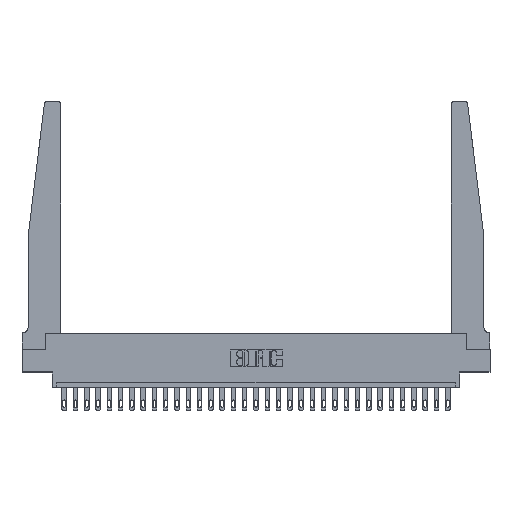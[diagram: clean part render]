
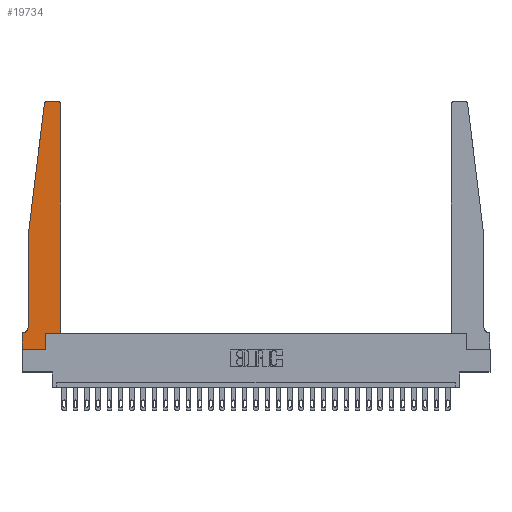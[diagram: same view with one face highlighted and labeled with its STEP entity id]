
A CAD part, top view. The second image highlights one B-rep face of the part: STEP entity #19734.
In plain terms, the highlighted planar face has unit normal (0, 0, 1).
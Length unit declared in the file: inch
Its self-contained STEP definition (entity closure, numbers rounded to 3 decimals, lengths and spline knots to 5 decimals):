
#332 = AXIS2_PLACEMENT_3D ( 'NONE', #8479, #10356, #16702 ) ;
#785 = CARTESIAN_POINT ( 'NONE',  ( 0.065, 1.25, 0.37 ) ) ;
#903 = EDGE_CURVE ( 'NONE', #14148, #15169, #9921, .T. ) ;
#911 = CARTESIAN_POINT ( 'NONE',  ( 0.425, 2.72, 0.37 ) ) ;
#1199 = CARTESIAN_POINT ( 'NONE',  ( 0.27653, 2.75, 0.37 ) ) ;
#1359 = DIRECTION ( 'NONE',  ( 1., 0., 0. ) ) ;
#1382 = EDGE_CURVE ( 'NONE', #12449, #16580, #6742, .T. ) ;
#1622 = DIRECTION ( 'NONE',  ( 0., 0., 1. ) ) ;
#1807 = VERTEX_POINT ( 'NONE', #20517 ) ;
#1962 = EDGE_CURVE ( 'NONE', #22270, #1807, #5115, .T. ) ;
#2154 = VECTOR ( 'NONE', #15964, 39.37008 ) ;
#2273 = ORIENTED_EDGE ( 'NONE', *, *, #1382, .T. ) ;
#2474 = ORIENTED_EDGE ( 'NONE', *, *, #8058, .T. ) ;
#4136 = ORIENTED_EDGE ( 'NONE', *, *, #1962, .T. ) ;
#4383 = CIRCLE ( 'NONE', #20116, 0.03 ) ;
#4385 = CARTESIAN_POINT ( 'NONE',  ( 0., 0., 0.37 ) ) ;
#4834 = DIRECTION ( 'NONE',  ( 0., 1., 0. ) ) ;
#4835 = EDGE_CURVE ( 'NONE', #16580, #5265, #23646, .T. ) ;
#4985 = LINE ( 'NONE', #22328, #2154 ) ;
#5115 = LINE ( 'NONE', #17779, #12883 ) ;
#5265 = VERTEX_POINT ( 'NONE', #21598 ) ;
#5268 = EDGE_CURVE ( 'NONE', #20338, #21790, #19469, .T. ) ;
#5649 = ORIENTED_EDGE ( 'NONE', *, *, #14068, .T. ) ;
#5724 = VECTOR ( 'NONE', #12333, 39.37008 ) ;
#5973 = CARTESIAN_POINT ( 'NONE',  ( 0.2605, 0.18, 0.37 ) ) ;
#6209 = EDGE_CURVE ( 'NONE', #15169, #20338, #26520, .T. ) ;
#6343 = VERTEX_POINT ( 'NONE', #12493 ) ;
#6569 = DIRECTION ( 'NONE',  ( 0., 0., -1. ) ) ;
#6597 = LINE ( 'NONE', #4385, #26924 ) ;
#6742 = LINE ( 'NONE', #19855, #12827 ) ;
#6837 = CARTESIAN_POINT ( 'NONE',  ( 0.2605, 0.18, 0.37 ) ) ;
#6905 = CARTESIAN_POINT ( 'NONE',  ( 0.425, 0.18, 0.37 ) ) ;
#7841 = AXIS2_PLACEMENT_3D ( 'NONE', #15561, #21630, #15148 ) ;
#8018 = EDGE_CURVE ( 'NONE', #21790, #12449, #4383, .T. ) ;
#8058 = EDGE_CURVE ( 'NONE', #6343, #22270, #10218, .T. ) ;
#8479 = CARTESIAN_POINT ( 'NONE',  ( 0., 0.1875, 0.37 ) ) ;
#8959 = CARTESIAN_POINT ( 'NONE',  ( 0.065, 1.25, 0.37 ) ) ;
#9529 = CARTESIAN_POINT ( 'NONE',  ( 0.2605, 0., 0.37 ) ) ;
#9921 = LINE ( 'NONE', #5973, #23645 ) ;
#10218 = LINE ( 'NONE', #14726, #5724 ) ;
#10356 = DIRECTION ( 'NONE',  ( 0., 0., 1. ) ) ;
#10429 = DIRECTION ( 'NONE',  ( -1., 0., 0. ) ) ;
#10695 = AXIS2_PLACEMENT_3D ( 'NONE', #25951, #6569, #10429 ) ;
#10801 = ORIENTED_EDGE ( 'NONE', *, *, #18381, .T. ) ;
#11397 = CARTESIAN_POINT ( 'NONE',  ( 0.425, 0.18, 0.37 ) ) ;
#11712 = CARTESIAN_POINT ( 'NONE',  ( 0., 0.1875, 0.37 ) ) ;
#11961 = ORIENTED_EDGE ( 'NONE', *, *, #20251, .T. ) ;
#12040 = CARTESIAN_POINT ( 'NONE',  ( 0.065, 0.2375, 0.37 ) ) ;
#12327 = DIRECTION ( 'NONE',  ( 0., 1., 0. ) ) ;
#12333 = DIRECTION ( 'NONE',  ( -1., 0., 0. ) ) ;
#12449 = VERTEX_POINT ( 'NONE', #26100 ) ;
#12493 = CARTESIAN_POINT ( 'NONE',  ( 0.015, 0.1875, 0.37 ) ) ;
#12827 = VECTOR ( 'NONE', #23981, 39.37008 ) ;
#12883 = VECTOR ( 'NONE', #26603, 39.37008 ) ;
#14068 = EDGE_CURVE ( 'NONE', #5265, #19494, #26510, .T. ) ;
#14148 = VERTEX_POINT ( 'NONE', #9529 ) ;
#14726 = CARTESIAN_POINT ( 'NONE',  ( 0.065, 0.1875, 0.37 ) ) ;
#15090 = DIRECTION ( 'NONE',  ( 1., 0., 0. ) ) ;
#15148 = DIRECTION ( 'NONE',  ( 1., 0., 0. ) ) ;
#15169 = VERTEX_POINT ( 'NONE', #6837 ) ;
#15561 = CARTESIAN_POINT ( 'NONE',  ( 0.27653, 2.72, 0.37 ) ) ;
#15609 = VERTEX_POINT ( 'NONE', #12040 ) ;
#15961 = VECTOR ( 'NONE', #4834, 39.37008 ) ;
#15964 = DIRECTION ( 'NONE',  ( 0., -1., 0. ) ) ;
#16554 = PLANE ( 'NONE',  #332 ) ;
#16580 = VERTEX_POINT ( 'NONE', #1199 ) ;
#16702 = DIRECTION ( 'NONE',  ( 1., 0., 0. ) ) ;
#17563 = DIRECTION ( 'NONE',  ( -0.122, -0.992, 0. ) ) ;
#17779 = CARTESIAN_POINT ( 'NONE',  ( 0., 0., 0.37 ) ) ;
#18136 = DIRECTION ( 'NONE',  ( 1., 0., 0. ) ) ;
#18381 = EDGE_CURVE ( 'NONE', #1807, #14148, #6597, .T. ) ;
#18793 = FACE_OUTER_BOUND ( 'NONE', #20952, .T. ) ;
#19469 = LINE ( 'NONE', #6905, #15961 ) ;
#19494 = VERTEX_POINT ( 'NONE', #785 ) ;
#19734 = ADVANCED_FACE ( 'NONE', ( #18793 ), #16554, .T. ) ;
#19855 = CARTESIAN_POINT ( 'NONE',  ( 0.25, 2.75, 0.37 ) ) ;
#19982 = EDGE_CURVE ( 'NONE', #19494, #15609, #4985, .T. ) ;
#20116 = AXIS2_PLACEMENT_3D ( 'NONE', #23077, #1622, #1359 ) ;
#20251 = EDGE_CURVE ( 'NONE', #15609, #6343, #26525, .T. ) ;
#20338 = VERTEX_POINT ( 'NONE', #11397 ) ;
#20517 = CARTESIAN_POINT ( 'NONE',  ( 0., 0., 0.37 ) ) ;
#20952 = EDGE_LOOP ( 'NONE', ( #2273, #23254, #5649, #25463, #11961, #2474, #4136, #10801, #27919, #24738, #26969, #25029 ) ) ;
#21598 = CARTESIAN_POINT ( 'NONE',  ( 0.24675, 2.72367, 0.37 ) ) ;
#21630 = DIRECTION ( 'NONE',  ( 0., 0., 1. ) ) ;
#21790 = VERTEX_POINT ( 'NONE', #911 ) ;
#22270 = VERTEX_POINT ( 'NONE', #11712 ) ;
#22328 = CARTESIAN_POINT ( 'NONE',  ( 0.065, 1.25, 0.37 ) ) ;
#23077 = CARTESIAN_POINT ( 'NONE',  ( 0.395, 2.72, 0.37 ) ) ;
#23254 = ORIENTED_EDGE ( 'NONE', *, *, #4835, .T. ) ;
#23645 = VECTOR ( 'NONE', #12327, 39.37008 ) ;
#23646 = CIRCLE ( 'NONE', #7841, 0.03 ) ;
#23981 = DIRECTION ( 'NONE',  ( -1., 0., 0. ) ) ;
#24370 = CARTESIAN_POINT ( 'NONE',  ( 0.425, 0.18, 0.37 ) ) ;
#24426 = VECTOR ( 'NONE', #17563, 39.37008 ) ;
#24581 = VECTOR ( 'NONE', #18136, 39.37008 ) ;
#24738 = ORIENTED_EDGE ( 'NONE', *, *, #6209, .T. ) ;
#25029 = ORIENTED_EDGE ( 'NONE', *, *, #8018, .T. ) ;
#25463 = ORIENTED_EDGE ( 'NONE', *, *, #19982, .T. ) ;
#25951 = CARTESIAN_POINT ( 'NONE',  ( 0.015, 0.2375, 0.37 ) ) ;
#26100 = CARTESIAN_POINT ( 'NONE',  ( 0.395, 2.75, 0.37 ) ) ;
#26510 = LINE ( 'NONE', #8959, #24426 ) ;
#26520 = LINE ( 'NONE', #24370, #24581 ) ;
#26525 = CIRCLE ( 'NONE', #10695, 0.05 ) ;
#26603 = DIRECTION ( 'NONE',  ( 0., -1., 0. ) ) ;
#26924 = VECTOR ( 'NONE', #15090, 39.37008 ) ;
#26969 = ORIENTED_EDGE ( 'NONE', *, *, #5268, .T. ) ;
#27919 = ORIENTED_EDGE ( 'NONE', *, *, #903, .T. ) ;
